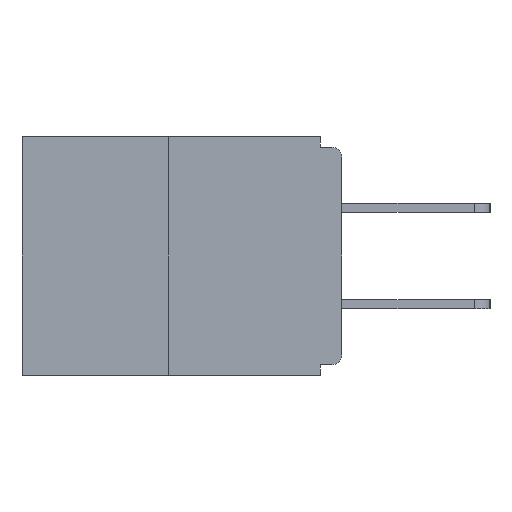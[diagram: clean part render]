
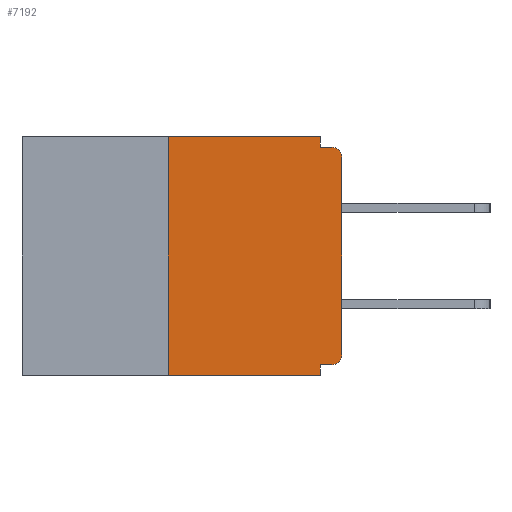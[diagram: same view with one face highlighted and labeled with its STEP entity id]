
A CAD part, left-side view. The second image highlights one B-rep face of the part: STEP entity #7192.
In plain terms, the highlighted planar face has unit normal (-1, 0, 0).
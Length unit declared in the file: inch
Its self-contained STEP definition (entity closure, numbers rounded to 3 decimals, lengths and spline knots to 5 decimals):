
#380 = CARTESIAN_POINT ( 'NONE',  ( 0., 0., -0.313 ) ) ;
#632 = CARTESIAN_POINT ( 'NONE',  ( 0., 0.031, -0.015 ) ) ;
#1578 = VERTEX_POINT ( 'NONE', #11927 ) ;
#1610 = LINE ( 'NONE', #3336, #14521 ) ;
#1626 = VERTEX_POINT ( 'NONE', #1884 ) ;
#1790 = LINE ( 'NONE', #14774, #14695 ) ;
#1815 = VECTOR ( 'NONE', #10120, 39.37008 ) ;
#1870 = VERTEX_POINT ( 'NONE', #8438 ) ;
#1884 = CARTESIAN_POINT ( 'NONE',  ( 0., 0.031, -0.343 ) ) ;
#1986 = DIRECTION ( 'NONE',  ( 0., 0., -1. ) ) ;
#2210 = CARTESIAN_POINT ( 'NONE',  ( 0., 0., 0. ) ) ;
#2568 = DIRECTION ( 'NONE',  ( 0., 1., 0. ) ) ;
#2589 = ORIENTED_EDGE ( 'NONE', *, *, #7968, .F. ) ;
#2637 = VECTOR ( 'NONE', #12419, 39.37008 ) ;
#3004 = DIRECTION ( 'NONE',  ( 0., 0., -1. ) ) ;
#3299 = EDGE_CURVE ( 'NONE', #8114, #1626, #10973, .T. ) ;
#3336 = CARTESIAN_POINT ( 'NONE',  ( 0., 0., -0.015 ) ) ;
#3455 = EDGE_CURVE ( 'NONE', #8184, #6227, #5431, .T. ) ;
#3558 = VECTOR ( 'NONE', #2568, 39.37008 ) ;
#4102 = EDGE_CURVE ( 'NONE', #7049, #9337, #1790, .T. ) ;
#4288 = LINE ( 'NONE', #10499, #3558 ) ;
#4465 = EDGE_LOOP ( 'NONE', ( #9148, #2589, #10328, #11593, #8795, #7367, #11447, #11116, #6760, #13050 ) ) ;
#4476 = CARTESIAN_POINT ( 'NONE',  ( 0., 0., -0.03 ) ) ;
#4663 = EDGE_CURVE ( 'NONE', #8676, #7909, #1610, .T. ) ;
#5215 = CIRCLE ( 'NONE', #14062, 0.015 ) ;
#5431 = LINE ( 'NONE', #2210, #1815 ) ;
#5495 = CIRCLE ( 'NONE', #8227, 0.015 ) ;
#5521 = DIRECTION ( 'NONE',  ( 1., 0., 0. ) ) ;
#5963 = LINE ( 'NONE', #14152, #12767 ) ;
#6168 = EDGE_CURVE ( 'NONE', #1870, #1626, #14808, .T. ) ;
#6227 = VERTEX_POINT ( 'NONE', #4476 ) ;
#6485 = CARTESIAN_POINT ( 'NONE',  ( 0., 0.015, -0.015 ) ) ;
#6719 = PLANE ( 'NONE',  #12237 ) ;
#6760 = ORIENTED_EDGE ( 'NONE', *, *, #4663, .F. ) ;
#6778 = EDGE_CURVE ( 'NONE', #1578, #8184, #5495, .T. ) ;
#6920 = CARTESIAN_POINT ( 'NONE',  ( 0., 0.031, -0.328 ) ) ;
#6923 = DIRECTION ( 'NONE',  ( -1., 0., 0. ) ) ;
#7049 = VERTEX_POINT ( 'NONE', #11722 ) ;
#7192 = ADVANCED_FACE ( 'NONE', ( #12465 ), #6719, .F. ) ;
#7339 = DIRECTION ( 'NONE',  ( 0., 0., -1. ) ) ;
#7367 = ORIENTED_EDGE ( 'NONE', *, *, #6778, .T. ) ;
#7598 = DIRECTION ( 'NONE',  ( 0., 0., 1. ) ) ;
#7909 = VERTEX_POINT ( 'NONE', #6485 ) ;
#7968 = EDGE_CURVE ( 'NONE', #1870, #7049, #11231, .T. ) ;
#8114 = VERTEX_POINT ( 'NONE', #6920 ) ;
#8184 = VERTEX_POINT ( 'NONE', #380 ) ;
#8227 = AXIS2_PLACEMENT_3D ( 'NONE', #13780, #6923, #9130 ) ;
#8438 = CARTESIAN_POINT ( 'NONE',  ( 0., 0.25, -0.343 ) ) ;
#8676 = VERTEX_POINT ( 'NONE', #632 ) ;
#8677 = VECTOR ( 'NONE', #3004, 39.37008 ) ;
#8795 = ORIENTED_EDGE ( 'NONE', *, *, #12079, .F. ) ;
#9130 = DIRECTION ( 'NONE',  ( 0., 0., -1. ) ) ;
#9148 = ORIENTED_EDGE ( 'NONE', *, *, #4102, .F. ) ;
#9337 = VERTEX_POINT ( 'NONE', #9559 ) ;
#9559 = CARTESIAN_POINT ( 'NONE',  ( 0., 0.031, 0. ) ) ;
#9767 = CARTESIAN_POINT ( 'NONE',  ( 0., 0.015, -0.03 ) ) ;
#10091 = EDGE_CURVE ( 'NONE', #9337, #8676, #5963, .T. ) ;
#10120 = DIRECTION ( 'NONE',  ( 0., 0., 1. ) ) ;
#10239 = DIRECTION ( 'NONE',  ( 0., -1., 0. ) ) ;
#10328 = ORIENTED_EDGE ( 'NONE', *, *, #6168, .T. ) ;
#10499 = CARTESIAN_POINT ( 'NONE',  ( 0., 0., -0.328 ) ) ;
#10973 = LINE ( 'NONE', #13041, #8677 ) ;
#11116 = ORIENTED_EDGE ( 'NONE', *, *, #14822, .T. ) ;
#11231 = LINE ( 'NONE', #13301, #14806 ) ;
#11447 = ORIENTED_EDGE ( 'NONE', *, *, #3455, .T. ) ;
#11593 = ORIENTED_EDGE ( 'NONE', *, *, #3299, .F. ) ;
#11722 = CARTESIAN_POINT ( 'NONE',  ( 0., 0.25, 0. ) ) ;
#11792 = DIRECTION ( 'NONE',  ( 0., 0., -1. ) ) ;
#11927 = CARTESIAN_POINT ( 'NONE',  ( 0., 0.015, -0.328 ) ) ;
#12079 = EDGE_CURVE ( 'NONE', #1578, #8114, #4288, .T. ) ;
#12237 = AXIS2_PLACEMENT_3D ( 'NONE', #14759, #5521, #1986 ) ;
#12373 = CARTESIAN_POINT ( 'NONE',  ( 0., 0.46, -0.343 ) ) ;
#12419 = DIRECTION ( 'NONE',  ( 0., -1., 0. ) ) ;
#12465 = FACE_OUTER_BOUND ( 'NONE', #4465, .T. ) ;
#12767 = VECTOR ( 'NONE', #11792, 39.37008 ) ;
#13041 = CARTESIAN_POINT ( 'NONE',  ( 0., 0.031, -0.343 ) ) ;
#13050 = ORIENTED_EDGE ( 'NONE', *, *, #10091, .F. ) ;
#13248 = DIRECTION ( 'NONE',  ( -1., 0., 0. ) ) ;
#13301 = CARTESIAN_POINT ( 'NONE',  ( 0., 0.25, 0. ) ) ;
#13642 = DIRECTION ( 'NONE',  ( 0., -1., 0. ) ) ;
#13780 = CARTESIAN_POINT ( 'NONE',  ( 0., 0.015, -0.313 ) ) ;
#14062 = AXIS2_PLACEMENT_3D ( 'NONE', #9767, #13248, #7339 ) ;
#14152 = CARTESIAN_POINT ( 'NONE',  ( 0., 0.031, 0. ) ) ;
#14521 = VECTOR ( 'NONE', #10239, 39.37008 ) ;
#14695 = VECTOR ( 'NONE', #13642, 39.37008 ) ;
#14759 = CARTESIAN_POINT ( 'NONE',  ( 0., 0.46, 0. ) ) ;
#14774 = CARTESIAN_POINT ( 'NONE',  ( 0., 0.46, 0. ) ) ;
#14806 = VECTOR ( 'NONE', #7598, 39.37008 ) ;
#14808 = LINE ( 'NONE', #12373, #2637 ) ;
#14822 = EDGE_CURVE ( 'NONE', #6227, #7909, #5215, .T. ) ;
